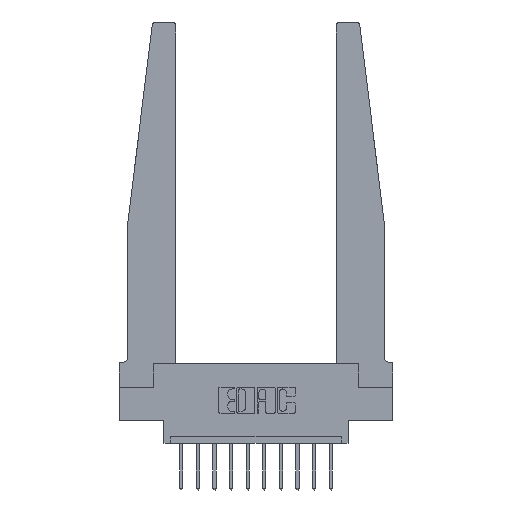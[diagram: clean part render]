
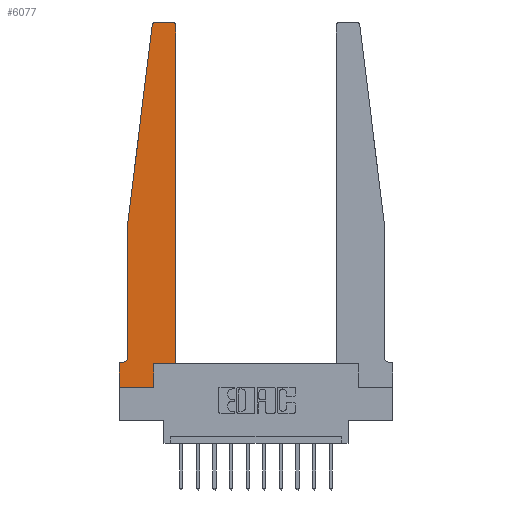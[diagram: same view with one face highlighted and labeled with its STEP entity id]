
A CAD part, top view. The second image highlights one B-rep face of the part: STEP entity #6077.
In plain terms, the highlighted planar face has unit normal (0, 0, 1).
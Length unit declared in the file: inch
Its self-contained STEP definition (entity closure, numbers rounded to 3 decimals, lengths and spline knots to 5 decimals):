
#63 = CARTESIAN_POINT ( 'NONE',  ( 0.065, 1.25, 0.37 ) ) ;
#449 = CARTESIAN_POINT ( 'NONE',  ( 0.425, 2.72, 0.37 ) ) ;
#483 = CARTESIAN_POINT ( 'NONE',  ( 0., 0., 0.37 ) ) ;
#645 = CARTESIAN_POINT ( 'NONE',  ( 0.065, 0.1875, 0.37 ) ) ;
#1296 = CARTESIAN_POINT ( 'NONE',  ( 0., 0.1875, 0.37 ) ) ;
#1532 = EDGE_CURVE ( 'NONE', #2370, #9911, #9543, .T. ) ;
#1616 = DIRECTION ( 'NONE',  ( 0., -1., 0. ) ) ;
#1979 = VECTOR ( 'NONE', #7637, 39.37008 ) ;
#2019 = AXIS2_PLACEMENT_3D ( 'NONE', #12386, #6401, #14771 ) ;
#2027 = ORIENTED_EDGE ( 'NONE', *, *, #12127, .T. ) ;
#2216 = EDGE_CURVE ( 'NONE', #14294, #13954, #10300, .T. ) ;
#2242 = DIRECTION ( 'NONE',  ( -1., 0., 0. ) ) ;
#2338 = CARTESIAN_POINT ( 'NONE',  ( 0.2605, 0.18, 0.37 ) ) ;
#2370 = VERTEX_POINT ( 'NONE', #4659 ) ;
#2380 = DIRECTION ( 'NONE',  ( -0.122, -0.992, 0. ) ) ;
#2386 = CARTESIAN_POINT ( 'NONE',  ( 0.25, 2.75, 0.37 ) ) ;
#2394 = AXIS2_PLACEMENT_3D ( 'NONE', #12165, #4993, #10931 ) ;
#2523 = CIRCLE ( 'NONE', #8190, 0.05 ) ;
#2557 = DIRECTION ( 'NONE',  ( 0., 0., -1. ) ) ;
#2634 = ORIENTED_EDGE ( 'NONE', *, *, #13139, .T. ) ;
#2694 = CIRCLE ( 'NONE', #2019, 0.03 ) ;
#3442 = VECTOR ( 'NONE', #5783, 39.37008 ) ;
#3795 = CARTESIAN_POINT ( 'NONE',  ( 0., 0., 0.37 ) ) ;
#4135 = ORIENTED_EDGE ( 'NONE', *, *, #8460, .T. ) ;
#4286 = ORIENTED_EDGE ( 'NONE', *, *, #7285, .T. ) ;
#4333 = DIRECTION ( 'NONE',  ( 1., 0., 0. ) ) ;
#4395 = LINE ( 'NONE', #4901, #12056 ) ;
#4430 = CARTESIAN_POINT ( 'NONE',  ( 0., 0.1875, 0.37 ) ) ;
#4659 = CARTESIAN_POINT ( 'NONE',  ( 0.015, 0.1875, 0.37 ) ) ;
#4901 = CARTESIAN_POINT ( 'NONE',  ( 0.2605, 0.18, 0.37 ) ) ;
#4993 = DIRECTION ( 'NONE',  ( 0., 0., 1. ) ) ;
#5625 = ORIENTED_EDGE ( 'NONE', *, *, #2216, .T. ) ;
#5783 = DIRECTION ( 'NONE',  ( 0., 1., 0. ) ) ;
#5788 = EDGE_CURVE ( 'NONE', #12095, #8668, #7984, .T. ) ;
#5981 = CARTESIAN_POINT ( 'NONE',  ( 0.425, 0.18, 0.37 ) ) ;
#5996 = CARTESIAN_POINT ( 'NONE',  ( 0.425, 0.18, 0.37 ) ) ;
#6002 = ORIENTED_EDGE ( 'NONE', *, *, #1532, .T. ) ;
#6066 = LINE ( 'NONE', #63, #12842 ) ;
#6077 = ADVANCED_FACE ( 'NONE', ( #8536 ), #9195, .T. ) ;
#6356 = VECTOR ( 'NONE', #2242, 39.37008 ) ;
#6371 = CARTESIAN_POINT ( 'NONE',  ( 0., 0., 0.37 ) ) ;
#6401 = DIRECTION ( 'NONE',  ( 0., 0., 1. ) ) ;
#6485 = EDGE_CURVE ( 'NONE', #15101, #14294, #6066, .T. ) ;
#6612 = LINE ( 'NONE', #6986, #3442 ) ;
#6694 = VECTOR ( 'NONE', #7947, 39.37008 ) ;
#6844 = VECTOR ( 'NONE', #9632, 39.37008 ) ;
#6891 = CARTESIAN_POINT ( 'NONE',  ( 0.2605, 0., 0.37 ) ) ;
#6905 = LINE ( 'NONE', #3795, #10330 ) ;
#6986 = CARTESIAN_POINT ( 'NONE',  ( 0.425, 0.18, 0.37 ) ) ;
#7078 = VERTEX_POINT ( 'NONE', #10486 ) ;
#7279 = EDGE_CURVE ( 'NONE', #12477, #12095, #4395, .T. ) ;
#7285 = EDGE_CURVE ( 'NONE', #13954, #2370, #2523, .T. ) ;
#7522 = EDGE_CURVE ( 'NONE', #7078, #15101, #2694, .T. ) ;
#7637 = DIRECTION ( 'NONE',  ( 1., 0., 0. ) ) ;
#7947 = DIRECTION ( 'NONE',  ( 0., -1., 0. ) ) ;
#7984 = LINE ( 'NONE', #5996, #6844 ) ;
#8096 = VERTEX_POINT ( 'NONE', #12041 ) ;
#8190 = AXIS2_PLACEMENT_3D ( 'NONE', #14469, #2557, #10941 ) ;
#8284 = EDGE_CURVE ( 'NONE', #10995, #12477, #11873, .T. ) ;
#8460 = EDGE_CURVE ( 'NONE', #8668, #9842, #6612, .T. ) ;
#8536 = FACE_OUTER_BOUND ( 'NONE', #13082, .T. ) ;
#8561 = ORIENTED_EDGE ( 'NONE', *, *, #8284, .T. ) ;
#8668 = VERTEX_POINT ( 'NONE', #5981 ) ;
#8995 = CARTESIAN_POINT ( 'NONE',  ( 0.065, 1.25, 0.37 ) ) ;
#9195 = PLANE ( 'NONE',  #9635 ) ;
#9543 = LINE ( 'NONE', #645, #13643 ) ;
#9632 = DIRECTION ( 'NONE',  ( 1., 0., 0. ) ) ;
#9635 = AXIS2_PLACEMENT_3D ( 'NONE', #4430, #11610, #4333 ) ;
#9842 = VERTEX_POINT ( 'NONE', #449 ) ;
#9911 = VERTEX_POINT ( 'NONE', #1296 ) ;
#10300 = LINE ( 'NONE', #8995, #6694 ) ;
#10330 = VECTOR ( 'NONE', #1616, 39.37008 ) ;
#10486 = CARTESIAN_POINT ( 'NONE',  ( 0.27653, 2.75, 0.37 ) ) ;
#10737 = ORIENTED_EDGE ( 'NONE', *, *, #6485, .T. ) ;
#10842 = CIRCLE ( 'NONE', #2394, 0.03 ) ;
#10931 = DIRECTION ( 'NONE',  ( 1., 0., 0. ) ) ;
#10941 = DIRECTION ( 'NONE',  ( -1., 0., 0. ) ) ;
#10995 = VERTEX_POINT ( 'NONE', #483 ) ;
#10999 = ORIENTED_EDGE ( 'NONE', *, *, #7279, .T. ) ;
#11610 = DIRECTION ( 'NONE',  ( 0., 0., 1. ) ) ;
#11873 = LINE ( 'NONE', #6371, #1979 ) ;
#12041 = CARTESIAN_POINT ( 'NONE',  ( 0.395, 2.75, 0.37 ) ) ;
#12056 = VECTOR ( 'NONE', #12075, 39.37008 ) ;
#12075 = DIRECTION ( 'NONE',  ( 0., 1., 0. ) ) ;
#12095 = VERTEX_POINT ( 'NONE', #2338 ) ;
#12127 = EDGE_CURVE ( 'NONE', #8096, #7078, #13304, .T. ) ;
#12165 = CARTESIAN_POINT ( 'NONE',  ( 0.395, 2.72, 0.37 ) ) ;
#12276 = ORIENTED_EDGE ( 'NONE', *, *, #5788, .T. ) ;
#12358 = ORIENTED_EDGE ( 'NONE', *, *, #7522, .T. ) ;
#12386 = CARTESIAN_POINT ( 'NONE',  ( 0.27653, 2.72, 0.37 ) ) ;
#12477 = VERTEX_POINT ( 'NONE', #6891 ) ;
#12678 = CARTESIAN_POINT ( 'NONE',  ( 0.24675, 2.72367, 0.37 ) ) ;
#12842 = VECTOR ( 'NONE', #2380, 39.37008 ) ;
#13082 = EDGE_LOOP ( 'NONE', ( #2027, #12358, #10737, #5625, #4286, #6002, #2634, #8561, #10999, #12276, #4135, #14666 ) ) ;
#13139 = EDGE_CURVE ( 'NONE', #9911, #10995, #6905, .T. ) ;
#13304 = LINE ( 'NONE', #2386, #6356 ) ;
#13643 = VECTOR ( 'NONE', #13765, 39.37008 ) ;
#13765 = DIRECTION ( 'NONE',  ( -1., 0., 0. ) ) ;
#13954 = VERTEX_POINT ( 'NONE', #15102 ) ;
#14294 = VERTEX_POINT ( 'NONE', #14362 ) ;
#14330 = EDGE_CURVE ( 'NONE', #9842, #8096, #10842, .T. ) ;
#14362 = CARTESIAN_POINT ( 'NONE',  ( 0.065, 1.25, 0.37 ) ) ;
#14469 = CARTESIAN_POINT ( 'NONE',  ( 0.015, 0.2375, 0.37 ) ) ;
#14666 = ORIENTED_EDGE ( 'NONE', *, *, #14330, .T. ) ;
#14771 = DIRECTION ( 'NONE',  ( 1., 0., 0. ) ) ;
#15101 = VERTEX_POINT ( 'NONE', #12678 ) ;
#15102 = CARTESIAN_POINT ( 'NONE',  ( 0.065, 0.2375, 0.37 ) ) ;
